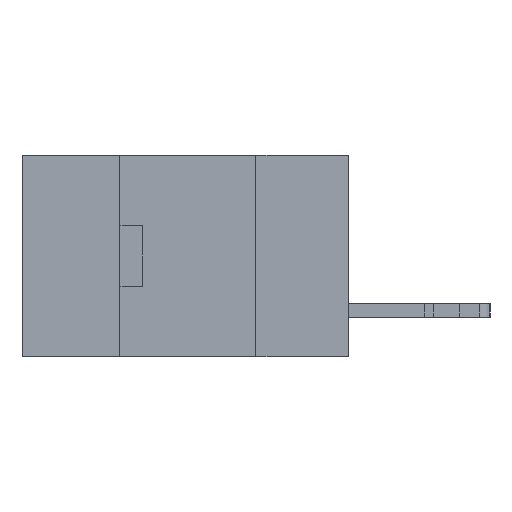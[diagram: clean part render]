
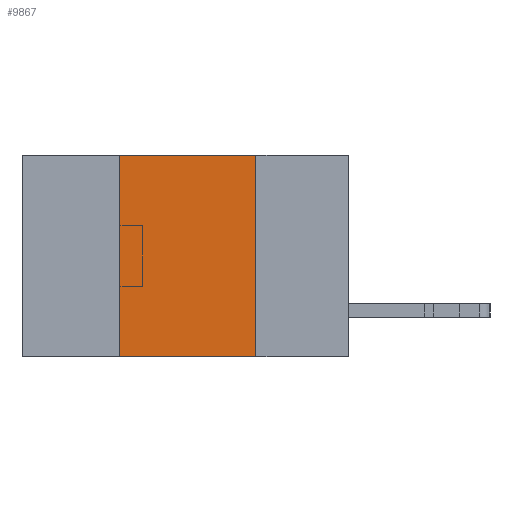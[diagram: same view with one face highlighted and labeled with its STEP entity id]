
A CAD part, left-side view. The second image highlights one B-rep face of the part: STEP entity #9867.
In plain terms, the highlighted planar face has unit normal (-1, 0, 0).
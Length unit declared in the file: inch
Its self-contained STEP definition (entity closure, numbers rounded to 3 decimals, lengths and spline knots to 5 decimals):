
#253 = VECTOR ( 'NONE', #13957, 39.37008 ) ;
#372 = LINE ( 'NONE', #14059, #11090 ) ;
#577 = DIRECTION ( 'NONE',  ( 0., 0., 1. ) ) ;
#2586 = ORIENTED_EDGE ( 'NONE', *, *, #15606, .F. ) ;
#2765 = EDGE_CURVE ( 'NONE', #17206, #7113, #372, .T. ) ;
#3492 = ORIENTED_EDGE ( 'NONE', *, *, #2765, .F. ) ;
#3966 = VERTEX_POINT ( 'NONE', #16975 ) ;
#4589 = VECTOR ( 'NONE', #14554, 39.37008 ) ;
#5920 = LINE ( 'NONE', #26500, #253 ) ;
#6914 = CARTESIAN_POINT ( 'NONE',  ( 0., 0.42, -0.37 ) ) ;
#7113 = VERTEX_POINT ( 'NONE', #15154 ) ;
#9287 = PLANE ( 'NONE',  #23538 ) ;
#9773 = EDGE_LOOP ( 'NONE', ( #3492, #17846, #2586, #18831 ) ) ;
#9867 = ADVANCED_FACE ( 'NONE', ( #26009 ), #9287, .F. ) ;
#10708 = LINE ( 'NONE', #6914, #15662 ) ;
#11090 = VECTOR ( 'NONE', #24500, 39.37008 ) ;
#11376 = EDGE_CURVE ( 'NONE', #3966, #17206, #15894, .T. ) ;
#11542 = CARTESIAN_POINT ( 'NONE',  ( 0., 0.6, 0. ) ) ;
#13667 = DIRECTION ( 'NONE',  ( 0., 0., -1. ) ) ;
#13957 = DIRECTION ( 'NONE',  ( 0., -1., 0. ) ) ;
#14059 = CARTESIAN_POINT ( 'NONE',  ( 0., 0.17, -0.37 ) ) ;
#14554 = DIRECTION ( 'NONE',  ( 0., -1., 0. ) ) ;
#15154 = CARTESIAN_POINT ( 'NONE',  ( 0., 0.17, -0.37 ) ) ;
#15606 = EDGE_CURVE ( 'NONE', #23046, #3966, #10708, .T. ) ;
#15662 = VECTOR ( 'NONE', #577, 39.37008 ) ;
#15894 = LINE ( 'NONE', #16670, #4589 ) ;
#16670 = CARTESIAN_POINT ( 'NONE',  ( 0., 0.6, 0. ) ) ;
#16975 = CARTESIAN_POINT ( 'NONE',  ( 0., 0.42, 0. ) ) ;
#17006 = EDGE_CURVE ( 'NONE', #23046, #7113, #5920, .T. ) ;
#17206 = VERTEX_POINT ( 'NONE', #27126 ) ;
#17846 = ORIENTED_EDGE ( 'NONE', *, *, #11376, .F. ) ;
#18831 = ORIENTED_EDGE ( 'NONE', *, *, #17006, .T. ) ;
#22983 = CARTESIAN_POINT ( 'NONE',  ( 0., 0.42, -0.37 ) ) ;
#23046 = VERTEX_POINT ( 'NONE', #22983 ) ;
#23538 = AXIS2_PLACEMENT_3D ( 'NONE', #11542, #26207, #13667 ) ;
#24500 = DIRECTION ( 'NONE',  ( 0., 0., -1. ) ) ;
#26009 = FACE_OUTER_BOUND ( 'NONE', #9773, .T. ) ;
#26207 = DIRECTION ( 'NONE',  ( 1., 0., 0. ) ) ;
#26500 = CARTESIAN_POINT ( 'NONE',  ( 0., 0.6, -0.37 ) ) ;
#27126 = CARTESIAN_POINT ( 'NONE',  ( 0., 0.17, 0. ) ) ;
